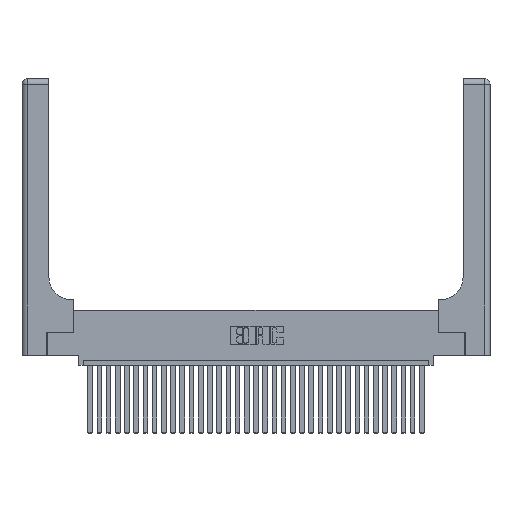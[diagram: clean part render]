
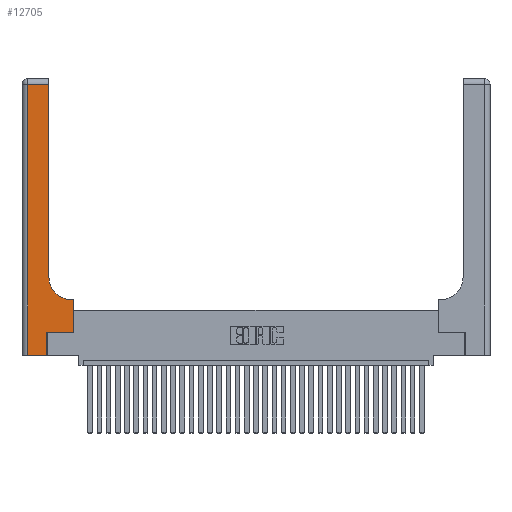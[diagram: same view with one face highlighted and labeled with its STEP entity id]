
A CAD part, top view. The second image highlights one B-rep face of the part: STEP entity #12705.
In plain terms, the highlighted planar face has unit normal (0, 0, 1).
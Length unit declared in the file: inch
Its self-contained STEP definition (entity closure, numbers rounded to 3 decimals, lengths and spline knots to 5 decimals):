
#449 = EDGE_CURVE ( 'NONE', #24972, #24423, #9943, .T. ) ;
#910 = EDGE_CURVE ( 'NONE', #11885, #1361, #2214, .T. ) ;
#1361 = VERTEX_POINT ( 'NONE', #8983 ) ;
#1385 = ORIENTED_EDGE ( 'NONE', *, *, #26422, .T. ) ;
#1450 = CARTESIAN_POINT ( 'NONE',  ( 0.5415, 0.85, 0.37 ) ) ;
#1609 = EDGE_CURVE ( 'NONE', #24423, #12678, #5896, .T. ) ;
#1932 = ORIENTED_EDGE ( 'NONE', *, *, #10616, .T. ) ;
#2038 = CARTESIAN_POINT ( 'NONE',  ( 0.269, 0.25, 0.37 ) ) ;
#2203 = DIRECTION ( 'NONE',  ( 0., 0., -1. ) ) ;
#2214 = LINE ( 'NONE', #24911, #30651 ) ;
#3175 = CARTESIAN_POINT ( 'NONE',  ( 0.06, 0., 0.37 ) ) ;
#4315 = CARTESIAN_POINT ( 'NONE',  ( 0.269, 0.25, 0.37 ) ) ;
#4409 = CARTESIAN_POINT ( 'NONE',  ( 0., 2.94, 0.37 ) ) ;
#5048 = CARTESIAN_POINT ( 'NONE',  ( 0., 0., 0.37 ) ) ;
#5694 = DIRECTION ( 'NONE',  ( -1., 0., 0. ) ) ;
#5896 = LINE ( 'NONE', #4409, #22594 ) ;
#6128 = CARTESIAN_POINT ( 'NONE',  ( 0.5415, 0.6, 0.37 ) ) ;
#6334 = DIRECTION ( 'NONE',  ( 1., 0., 0. ) ) ;
#6637 = VECTOR ( 'NONE', #5694, 39.37008 ) ;
#6682 = DIRECTION ( 'NONE',  ( -1., 0., 0. ) ) ;
#7040 = ORIENTED_EDGE ( 'NONE', *, *, #28089, .T. ) ;
#7169 = PLANE ( 'NONE',  #9830 ) ;
#8983 = CARTESIAN_POINT ( 'NONE',  ( 0.5585, 0.6, 0.37 ) ) ;
#9237 = EDGE_CURVE ( 'NONE', #31196, #20691, #31989, .T. ) ;
#9830 = AXIS2_PLACEMENT_3D ( 'NONE', #15006, #14896, #19690 ) ;
#9943 = LINE ( 'NONE', #23588, #16054 ) ;
#10255 = DIRECTION ( 'NONE',  ( 0., -1., 0. ) ) ;
#10598 = CARTESIAN_POINT ( 'NONE',  ( 0.269, 0., 0.37 ) ) ;
#10616 = EDGE_CURVE ( 'NONE', #20691, #11885, #18979, .T. ) ;
#11519 = LINE ( 'NONE', #5048, #23723 ) ;
#11885 = VERTEX_POINT ( 'NONE', #22863 ) ;
#12414 = CARTESIAN_POINT ( 'NONE',  ( 0.06, 3., 0.37 ) ) ;
#12678 = VERTEX_POINT ( 'NONE', #22307 ) ;
#12705 = ADVANCED_FACE ( 'NONE', ( #13933 ), #7169, .F. ) ;
#13244 = DIRECTION ( 'NONE',  ( 0., 1., 0. ) ) ;
#13933 = FACE_OUTER_BOUND ( 'NONE', #28727, .T. ) ;
#14746 = CIRCLE ( 'NONE', #27252, 0.25 ) ;
#14896 = DIRECTION ( 'NONE',  ( 0., 0., -1. ) ) ;
#15006 = CARTESIAN_POINT ( 'NONE',  ( 0., 3., 0.37 ) ) ;
#15361 = VECTOR ( 'NONE', #10255, 39.37008 ) ;
#15721 = VECTOR ( 'NONE', #30872, 39.37008 ) ;
#15831 = VERTEX_POINT ( 'NONE', #6128 ) ;
#16005 = LINE ( 'NONE', #28885, #6637 ) ;
#16054 = VECTOR ( 'NONE', #13244, 39.37008 ) ;
#16698 = DIRECTION ( 'NONE',  ( 0., 1., 0. ) ) ;
#17031 = ORIENTED_EDGE ( 'NONE', *, *, #449, .T. ) ;
#18979 = LINE ( 'NONE', #2038, #15721 ) ;
#19004 = VECTOR ( 'NONE', #16698, 39.37008 ) ;
#19690 = DIRECTION ( 'NONE',  ( -1., 0., 0. ) ) ;
#20691 = VERTEX_POINT ( 'NONE', #4315 ) ;
#20870 = CARTESIAN_POINT ( 'NONE',  ( 0.2915, 2.94, 0.37 ) ) ;
#21846 = CARTESIAN_POINT ( 'NONE',  ( 0.2915, 0.85, 0.37 ) ) ;
#22186 = ORIENTED_EDGE ( 'NONE', *, *, #1609, .T. ) ;
#22307 = CARTESIAN_POINT ( 'NONE',  ( 0.06, 2.94, 0.37 ) ) ;
#22594 = VECTOR ( 'NONE', #6682, 39.37008 ) ;
#22863 = CARTESIAN_POINT ( 'NONE',  ( 0.5585, 0.25, 0.37 ) ) ;
#23588 = CARTESIAN_POINT ( 'NONE',  ( 0.2915, 3., 0.37 ) ) ;
#23723 = VECTOR ( 'NONE', #28333, 39.37008 ) ;
#23881 = EDGE_CURVE ( 'NONE', #15831, #24972, #14746, .T. ) ;
#24380 = ORIENTED_EDGE ( 'NONE', *, *, #910, .T. ) ;
#24423 = VERTEX_POINT ( 'NONE', #20870 ) ;
#24911 = CARTESIAN_POINT ( 'NONE',  ( 0.5585, 0.25, 0.37 ) ) ;
#24972 = VERTEX_POINT ( 'NONE', #21846 ) ;
#25777 = ORIENTED_EDGE ( 'NONE', *, *, #9237, .T. ) ;
#26422 = EDGE_CURVE ( 'NONE', #12678, #28610, #32019, .T. ) ;
#27251 = ORIENTED_EDGE ( 'NONE', *, *, #27940, .T. ) ;
#27252 = AXIS2_PLACEMENT_3D ( 'NONE', #1450, #2203, #6334 ) ;
#27940 = EDGE_CURVE ( 'NONE', #28610, #31196, #11519, .T. ) ;
#28089 = EDGE_CURVE ( 'NONE', #1361, #15831, #16005, .T. ) ;
#28333 = DIRECTION ( 'NONE',  ( 1., 0., 0. ) ) ;
#28610 = VERTEX_POINT ( 'NONE', #3175 ) ;
#28727 = EDGE_LOOP ( 'NONE', ( #17031, #22186, #1385, #27251, #25777, #1932, #24380, #7040, #30341 ) ) ;
#28885 = CARTESIAN_POINT ( 'NONE',  ( 0.2915, 0.6, 0.37 ) ) ;
#30324 = DIRECTION ( 'NONE',  ( 0., 1., 0. ) ) ;
#30341 = ORIENTED_EDGE ( 'NONE', *, *, #23881, .T. ) ;
#30651 = VECTOR ( 'NONE', #30324, 39.37008 ) ;
#30872 = DIRECTION ( 'NONE',  ( 1., 0., 0. ) ) ;
#31196 = VERTEX_POINT ( 'NONE', #10598 ) ;
#31989 = LINE ( 'NONE', #32258, #19004 ) ;
#32019 = LINE ( 'NONE', #12414, #15361 ) ;
#32258 = CARTESIAN_POINT ( 'NONE',  ( 0.269, 0., 0.37 ) ) ;
